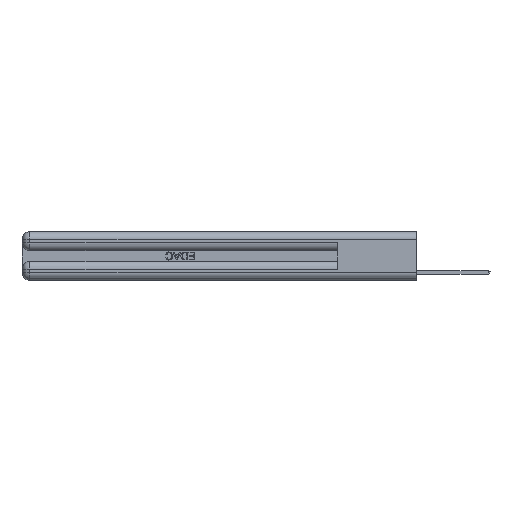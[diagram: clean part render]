
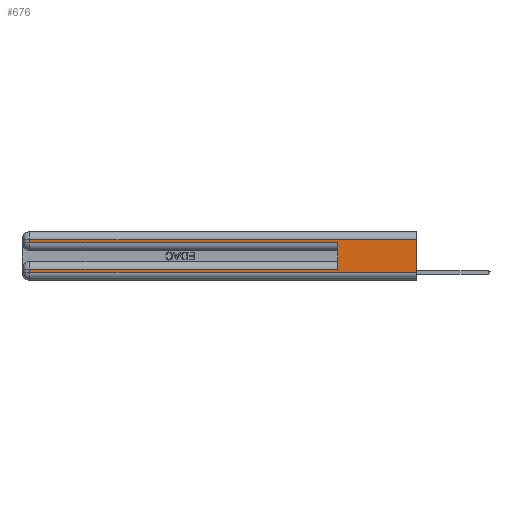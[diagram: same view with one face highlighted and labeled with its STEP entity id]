
A CAD part, left-side view. The second image highlights one B-rep face of the part: STEP entity #676.
In plain terms, the highlighted planar face has unit normal (-1, 0, 0).
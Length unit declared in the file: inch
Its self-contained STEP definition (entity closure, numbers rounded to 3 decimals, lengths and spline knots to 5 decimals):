
#676 = ADVANCED_FACE ( 'NONE', ( #23083 ), #33807, .F. ) ;
#1160 = DIRECTION ( 'NONE',  ( 0., 1., 0. ) ) ;
#2173 = CARTESIAN_POINT ( 'NONE',  ( 0., 0., 0.37 ) ) ;
#2580 = ORIENTED_EDGE ( 'NONE', *, *, #21133, .T. ) ;
#2691 = EDGE_CURVE ( 'NONE', #7888, #31047, #27550, .T. ) ;
#2898 = LINE ( 'NONE', #18590, #11220 ) ;
#3788 = CARTESIAN_POINT ( 'NONE',  ( 0., 0., 0.06 ) ) ;
#3795 = LINE ( 'NONE', #13208, #17086 ) ;
#4047 = LINE ( 'NONE', #14922, #9454 ) ;
#4211 = ORIENTED_EDGE ( 'NONE', *, *, #26732, .F. ) ;
#4522 = CARTESIAN_POINT ( 'NONE',  ( 0., 2.94, 0.285 ) ) ;
#6653 = EDGE_CURVE ( 'NONE', #34026, #12622, #16493, .T. ) ;
#6702 = EDGE_CURVE ( 'NONE', #7888, #8094, #4047, .T. ) ;
#7888 = VERTEX_POINT ( 'NONE', #19611 ) ;
#8054 = DIRECTION ( 'NONE',  ( 0., 0., 1. ) ) ;
#8094 = VERTEX_POINT ( 'NONE', #24294 ) ;
#8501 = CARTESIAN_POINT ( 'NONE',  ( 0., 0.6, 0.145 ) ) ;
#9454 = VECTOR ( 'NONE', #17458, 39.37008 ) ;
#9613 = DIRECTION ( 'NONE',  ( 0., 0., -1. ) ) ;
#9855 = ORIENTED_EDGE ( 'NONE', *, *, #25873, .T. ) ;
#10347 = VERTEX_POINT ( 'NONE', #25073 ) ;
#10678 = VECTOR ( 'NONE', #25492, 39.37008 ) ;
#11022 = ORIENTED_EDGE ( 'NONE', *, *, #6702, .T. ) ;
#11220 = VECTOR ( 'NONE', #32179, 39.37008 ) ;
#11919 = CARTESIAN_POINT ( 'NONE',  ( 0., 0., 0.31 ) ) ;
#12622 = VERTEX_POINT ( 'NONE', #24107 ) ;
#13208 = CARTESIAN_POINT ( 'NONE',  ( 0., 2.94, 0.37 ) ) ;
#13913 = ORIENTED_EDGE ( 'NONE', *, *, #22475, .T. ) ;
#14188 = DIRECTION ( 'NONE',  ( 0., 0., -1. ) ) ;
#14914 = CARTESIAN_POINT ( 'NONE',  ( 0., 0., 0.37 ) ) ;
#14922 = CARTESIAN_POINT ( 'NONE',  ( 0., 0., 0.085 ) ) ;
#15263 = VECTOR ( 'NONE', #1160, 39.37008 ) ;
#16343 = CARTESIAN_POINT ( 'NONE',  ( 0., 0., 0.06 ) ) ;
#16493 = LINE ( 'NONE', #11919, #15263 ) ;
#17086 = VECTOR ( 'NONE', #28793, 39.37008 ) ;
#17458 = DIRECTION ( 'NONE',  ( 0., 1., 0. ) ) ;
#17617 = ORIENTED_EDGE ( 'NONE', *, *, #2691, .F. ) ;
#18590 = CARTESIAN_POINT ( 'NONE',  ( 0., 0., 0.285 ) ) ;
#19479 = EDGE_CURVE ( 'NONE', #27392, #31047, #2898, .T. ) ;
#19611 = CARTESIAN_POINT ( 'NONE',  ( 0., 0.6, 0.085 ) ) ;
#20809 = EDGE_LOOP ( 'NONE', ( #4211, #30655, #9855, #23104, #17617, #11022, #13913, #2580 ) ) ;
#21133 = EDGE_CURVE ( 'NONE', #10347, #28549, #23302, .T. ) ;
#22475 = EDGE_CURVE ( 'NONE', #8094, #10347, #3795, .T. ) ;
#22953 = DIRECTION ( 'NONE',  ( 0., -1., 0. ) ) ;
#23057 = LINE ( 'NONE', #14914, #10678 ) ;
#23076 = DIRECTION ( 'NONE',  ( 1., 0., 0. ) ) ;
#23083 = FACE_OUTER_BOUND ( 'NONE', #20809, .T. ) ;
#23104 = ORIENTED_EDGE ( 'NONE', *, *, #19479, .T. ) ;
#23302 = LINE ( 'NONE', #3788, #23751 ) ;
#23657 = CARTESIAN_POINT ( 'NONE',  ( 0., 0.6, 0.285 ) ) ;
#23751 = VECTOR ( 'NONE', #22953, 39.37008 ) ;
#24107 = CARTESIAN_POINT ( 'NONE',  ( 0., 2.94, 0.31 ) ) ;
#24294 = CARTESIAN_POINT ( 'NONE',  ( 0., 2.94, 0.085 ) ) ;
#24433 = AXIS2_PLACEMENT_3D ( 'NONE', #2173, #23076, #9613 ) ;
#25073 = CARTESIAN_POINT ( 'NONE',  ( 0., 2.94, 0.06 ) ) ;
#25492 = DIRECTION ( 'NONE',  ( 0., 0., -1. ) ) ;
#25873 = EDGE_CURVE ( 'NONE', #12622, #27392, #33720, .T. ) ;
#26714 = VECTOR ( 'NONE', #14188, 39.37008 ) ;
#26732 = EDGE_CURVE ( 'NONE', #34026, #28549, #23057, .T. ) ;
#27392 = VERTEX_POINT ( 'NONE', #4522 ) ;
#27550 = LINE ( 'NONE', #8501, #28806 ) ;
#28549 = VERTEX_POINT ( 'NONE', #16343 ) ;
#28793 = DIRECTION ( 'NONE',  ( 0., 0., -1. ) ) ;
#28806 = VECTOR ( 'NONE', #8054, 39.37008 ) ;
#30655 = ORIENTED_EDGE ( 'NONE', *, *, #6653, .T. ) ;
#31047 = VERTEX_POINT ( 'NONE', #23657 ) ;
#32179 = DIRECTION ( 'NONE',  ( 0., -1., 0. ) ) ;
#32268 = CARTESIAN_POINT ( 'NONE',  ( 0., 2.94, 0.37 ) ) ;
#33720 = LINE ( 'NONE', #32268, #26714 ) ;
#33737 = CARTESIAN_POINT ( 'NONE',  ( 0., 0., 0.31 ) ) ;
#33807 = PLANE ( 'NONE',  #24433 ) ;
#34026 = VERTEX_POINT ( 'NONE', #33737 ) ;
